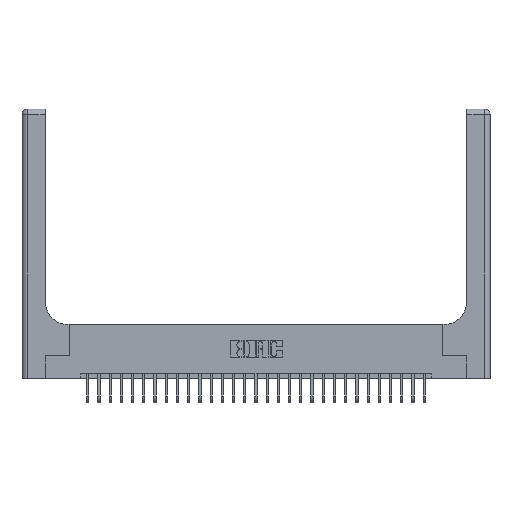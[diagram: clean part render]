
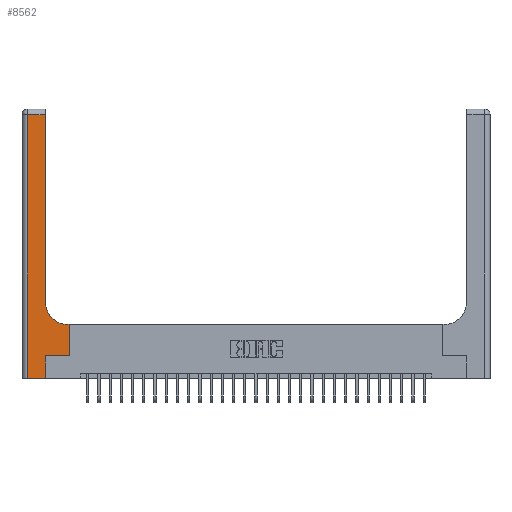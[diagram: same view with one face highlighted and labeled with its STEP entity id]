
A CAD part, top view. The second image highlights one B-rep face of the part: STEP entity #8562.
In plain terms, the highlighted planar face has unit normal (0, 0, 1).
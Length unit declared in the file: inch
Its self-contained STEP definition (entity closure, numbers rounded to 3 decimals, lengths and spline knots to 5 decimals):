
#49 = VERTEX_POINT ( 'NONE', #11362 ) ;
#771 = ORIENTED_EDGE ( 'NONE', *, *, #14230, .T. ) ;
#1462 = PLANE ( 'NONE',  #5094 ) ;
#1668 = CARTESIAN_POINT ( 'NONE',  ( 0., 2.94, 0.37 ) ) ;
#1733 = DIRECTION ( 'NONE',  ( 1., 0., 0. ) ) ;
#2953 = DIRECTION ( 'NONE',  ( 0., -1., 0. ) ) ;
#3729 = CARTESIAN_POINT ( 'NONE',  ( 0.51, 0.6, 0.37 ) ) ;
#4206 = VERTEX_POINT ( 'NONE', #8728 ) ;
#4715 = CARTESIAN_POINT ( 'NONE',  ( 0.265, 0., 0.37 ) ) ;
#5094 = AXIS2_PLACEMENT_3D ( 'NONE', #25483, #21514, #15601 ) ;
#5385 = CARTESIAN_POINT ( 'NONE',  ( 0.26, 3., 0.37 ) ) ;
#6431 = ORIENTED_EDGE ( 'NONE', *, *, #10095, .T. ) ;
#6855 = CARTESIAN_POINT ( 'NONE',  ( 0.528, 0.6, 0.37 ) ) ;
#7317 = CARTESIAN_POINT ( 'NONE',  ( 0.528, 0.25, 0.37 ) ) ;
#7611 = EDGE_LOOP ( 'NONE', ( #16875, #24845, #6431, #16293, #13137, #771, #12908, #10069, #7874 ) ) ;
#7637 = VECTOR ( 'NONE', #17200, 39.37008 ) ;
#7681 = VECTOR ( 'NONE', #17309, 39.37008 ) ;
#7874 = ORIENTED_EDGE ( 'NONE', *, *, #10140, .T. ) ;
#7970 = VECTOR ( 'NONE', #1733, 39.37008 ) ;
#8302 = VERTEX_POINT ( 'NONE', #4715 ) ;
#8323 = VERTEX_POINT ( 'NONE', #6855 ) ;
#8562 = ADVANCED_FACE ( 'NONE', ( #14154 ), #1462, .F. ) ;
#8728 = CARTESIAN_POINT ( 'NONE',  ( 0.26, 2.94, 0.37 ) ) ;
#9065 = CIRCLE ( 'NONE', #17909, 0.25 ) ;
#10069 = ORIENTED_EDGE ( 'NONE', *, *, #25967, .T. ) ;
#10095 = EDGE_CURVE ( 'NONE', #23023, #13434, #20932, .T. ) ;
#10140 = EDGE_CURVE ( 'NONE', #16789, #25491, #9065, .T. ) ;
#10959 = VERTEX_POINT ( 'NONE', #11941 ) ;
#11166 = LINE ( 'NONE', #12694, #16495 ) ;
#11188 = DIRECTION ( 'NONE',  ( 0., 0., -1. ) ) ;
#11362 = CARTESIAN_POINT ( 'NONE',  ( 0.265, 0.25, 0.37 ) ) ;
#11941 = CARTESIAN_POINT ( 'NONE',  ( 0.528, 0.25, 0.37 ) ) ;
#12694 = CARTESIAN_POINT ( 'NONE',  ( 0.265, 0., 0.37 ) ) ;
#12908 = ORIENTED_EDGE ( 'NONE', *, *, #14795, .T. ) ;
#12960 = LINE ( 'NONE', #25076, #7637 ) ;
#12994 = LINE ( 'NONE', #7317, #7681 ) ;
#13137 = ORIENTED_EDGE ( 'NONE', *, *, #13926, .T. ) ;
#13434 = VERTEX_POINT ( 'NONE', #25156 ) ;
#13521 = CARTESIAN_POINT ( 'NONE',  ( 0.26, 0.85, 0.37 ) ) ;
#13642 = LINE ( 'NONE', #1668, #23599 ) ;
#13916 = LINE ( 'NONE', #17880, #7970 ) ;
#13926 = EDGE_CURVE ( 'NONE', #8302, #49, #11166, .T. ) ;
#14154 = FACE_OUTER_BOUND ( 'NONE', #7611, .T. ) ;
#14230 = EDGE_CURVE ( 'NONE', #49, #10959, #14897, .T. ) ;
#14795 = EDGE_CURVE ( 'NONE', #10959, #8323, #12994, .T. ) ;
#14897 = LINE ( 'NONE', #15574, #19585 ) ;
#15574 = CARTESIAN_POINT ( 'NONE',  ( 0.265, 0.25, 0.37 ) ) ;
#15601 = DIRECTION ( 'NONE',  ( -1., 0., 0. ) ) ;
#15647 = VECTOR ( 'NONE', #2953, 39.37008 ) ;
#16293 = ORIENTED_EDGE ( 'NONE', *, *, #19641, .T. ) ;
#16495 = VECTOR ( 'NONE', #24626, 39.37008 ) ;
#16789 = VERTEX_POINT ( 'NONE', #3729 ) ;
#16875 = ORIENTED_EDGE ( 'NONE', *, *, #18167, .T. ) ;
#17200 = DIRECTION ( 'NONE',  ( -1., 0., 0. ) ) ;
#17309 = DIRECTION ( 'NONE',  ( 0., 1., 0. ) ) ;
#17427 = DIRECTION ( 'NONE',  ( 0., 1., 0. ) ) ;
#17824 = DIRECTION ( 'NONE',  ( -1., 0., 0. ) ) ;
#17880 = CARTESIAN_POINT ( 'NONE',  ( 0., 0., 0.37 ) ) ;
#17909 = AXIS2_PLACEMENT_3D ( 'NONE', #23136, #11188, #25108 ) ;
#18167 = EDGE_CURVE ( 'NONE', #25491, #4206, #18449, .T. ) ;
#18449 = LINE ( 'NONE', #5385, #23105 ) ;
#18986 = EDGE_CURVE ( 'NONE', #4206, #23023, #13642, .T. ) ;
#19583 = DIRECTION ( 'NONE',  ( 1., 0., 0. ) ) ;
#19585 = VECTOR ( 'NONE', #19583, 39.37008 ) ;
#19641 = EDGE_CURVE ( 'NONE', #13434, #8302, #13916, .T. ) ;
#20932 = LINE ( 'NONE', #24944, #15647 ) ;
#21217 = CARTESIAN_POINT ( 'NONE',  ( 0.06, 2.94, 0.37 ) ) ;
#21514 = DIRECTION ( 'NONE',  ( 0., 0., -1. ) ) ;
#23023 = VERTEX_POINT ( 'NONE', #21217 ) ;
#23105 = VECTOR ( 'NONE', #17427, 39.37008 ) ;
#23136 = CARTESIAN_POINT ( 'NONE',  ( 0.51, 0.85, 0.37 ) ) ;
#23599 = VECTOR ( 'NONE', #17824, 39.37008 ) ;
#24626 = DIRECTION ( 'NONE',  ( 0., 1., 0. ) ) ;
#24845 = ORIENTED_EDGE ( 'NONE', *, *, #18986, .T. ) ;
#24944 = CARTESIAN_POINT ( 'NONE',  ( 0.06, 3., 0.37 ) ) ;
#25076 = CARTESIAN_POINT ( 'NONE',  ( 0.26, 0.6, 0.37 ) ) ;
#25108 = DIRECTION ( 'NONE',  ( 1., 0., 0. ) ) ;
#25156 = CARTESIAN_POINT ( 'NONE',  ( 0.06, 0., 0.37 ) ) ;
#25483 = CARTESIAN_POINT ( 'NONE',  ( 0., 3., 0.37 ) ) ;
#25491 = VERTEX_POINT ( 'NONE', #13521 ) ;
#25967 = EDGE_CURVE ( 'NONE', #8323, #16789, #12960, .T. ) ;
